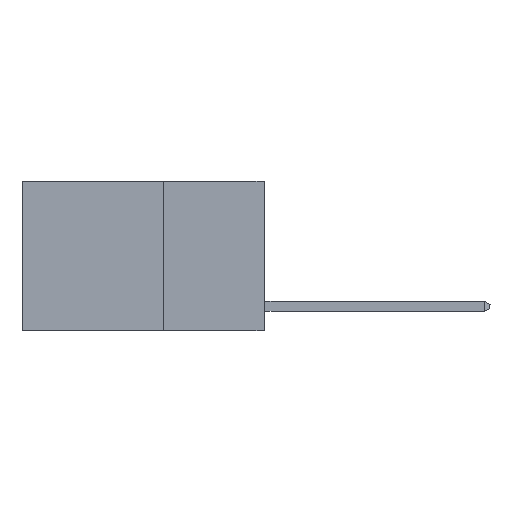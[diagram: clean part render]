
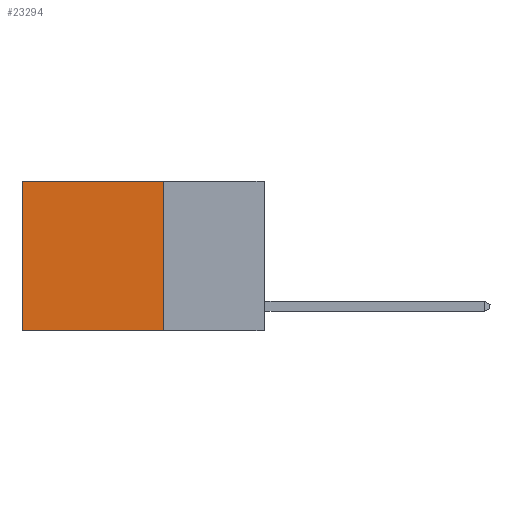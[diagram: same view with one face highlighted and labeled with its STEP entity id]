
A CAD part, left-side view. The second image highlights one B-rep face of the part: STEP entity #23294.
In plain terms, the highlighted planar face has unit normal (-1, 0, 0).
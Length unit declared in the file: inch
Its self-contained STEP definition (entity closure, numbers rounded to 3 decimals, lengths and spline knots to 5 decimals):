
#1845 = DIRECTION ( 'NONE',  ( 1., 0., 0. ) ) ;
#2290 = ORIENTED_EDGE ( 'NONE', *, *, #20375, .F. ) ;
#2298 = VECTOR ( 'NONE', #2481, 39.37008 ) ;
#2481 = DIRECTION ( 'NONE',  ( 0., 0., -1. ) ) ;
#3205 = AXIS2_PLACEMENT_3D ( 'NONE', #8129, #1845, #16567 ) ;
#3275 = EDGE_CURVE ( 'NONE', #3677, #23448, #18857, .T. ) ;
#3677 = VERTEX_POINT ( 'NONE', #9687 ) ;
#4041 = VECTOR ( 'NONE', #21681, 39.37008 ) ;
#4153 = LINE ( 'NONE', #21073, #8420 ) ;
#6202 = CARTESIAN_POINT ( 'NONE',  ( 0.2625, 0.6, 0. ) ) ;
#7866 = FACE_OUTER_BOUND ( 'NONE', #25320, .T. ) ;
#7967 = ORIENTED_EDGE ( 'NONE', *, *, #11048, .T. ) ;
#8129 = CARTESIAN_POINT ( 'NONE',  ( 0.2625, 0.25, 0. ) ) ;
#8420 = VECTOR ( 'NONE', #10688, 39.37008 ) ;
#8852 = CARTESIAN_POINT ( 'NONE',  ( 0.2625, 0.25, 0. ) ) ;
#8964 = VERTEX_POINT ( 'NONE', #22431 ) ;
#9194 = CARTESIAN_POINT ( 'NONE',  ( 0.2625, 0.25, 0. ) ) ;
#9687 = CARTESIAN_POINT ( 'NONE',  ( 0.2625, 0.6, 0. ) ) ;
#10262 = PLANE ( 'NONE',  #3205 ) ;
#10688 = DIRECTION ( 'NONE',  ( 0., 1., 0. ) ) ;
#10710 = CARTESIAN_POINT ( 'NONE',  ( 0.2625, 0.6, -0.37 ) ) ;
#11048 = EDGE_CURVE ( 'NONE', #26977, #3677, #15204, .T. ) ;
#14710 = EDGE_CURVE ( 'NONE', #26977, #8964, #24523, .T. ) ;
#15063 = CARTESIAN_POINT ( 'NONE',  ( 0.2625, 0.25, 0. ) ) ;
#15204 = LINE ( 'NONE', #9194, #4041 ) ;
#16567 = DIRECTION ( 'NONE',  ( 0., 0., -1. ) ) ;
#17616 = ORIENTED_EDGE ( 'NONE', *, *, #3275, .T. ) ;
#18857 = LINE ( 'NONE', #6202, #19501 ) ;
#19501 = VECTOR ( 'NONE', #26958, 39.37008 ) ;
#20375 = EDGE_CURVE ( 'NONE', #8964, #23448, #4153, .T. ) ;
#21073 = CARTESIAN_POINT ( 'NONE',  ( 0.2625, 0.25, -0.37 ) ) ;
#21681 = DIRECTION ( 'NONE',  ( 0., 1., 0. ) ) ;
#22431 = CARTESIAN_POINT ( 'NONE',  ( 0.2625, 0.25, -0.37 ) ) ;
#23294 = ADVANCED_FACE ( 'NONE', ( #7866 ), #10262, .F. ) ;
#23448 = VERTEX_POINT ( 'NONE', #10710 ) ;
#23537 = ORIENTED_EDGE ( 'NONE', *, *, #14710, .F. ) ;
#24523 = LINE ( 'NONE', #8852, #2298 ) ;
#25320 = EDGE_LOOP ( 'NONE', ( #17616, #2290, #23537, #7967 ) ) ;
#26958 = DIRECTION ( 'NONE',  ( 0., 0., -1. ) ) ;
#26977 = VERTEX_POINT ( 'NONE', #15063 ) ;
